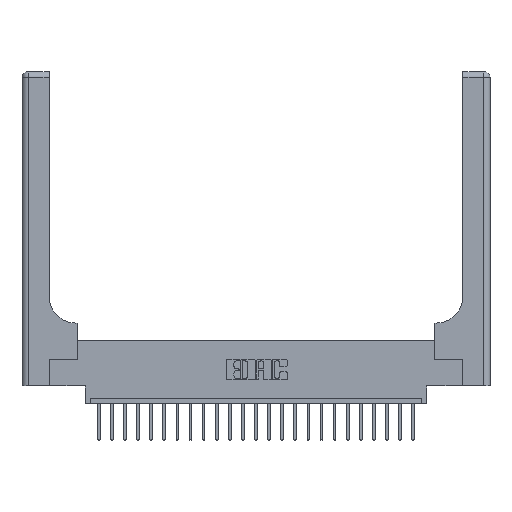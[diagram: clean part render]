
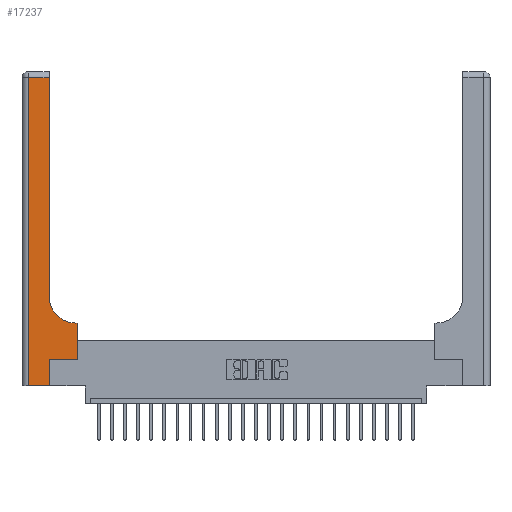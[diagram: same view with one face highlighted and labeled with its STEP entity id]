
A CAD part, top view. The second image highlights one B-rep face of the part: STEP entity #17237.
In plain terms, the highlighted planar face has unit normal (0, 0, 1).
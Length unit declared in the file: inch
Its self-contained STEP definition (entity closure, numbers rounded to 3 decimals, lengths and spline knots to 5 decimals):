
#562 = VERTEX_POINT ( 'NONE', #19831 ) ;
#1070 = DIRECTION ( 'NONE',  ( 0., 0., -1. ) ) ;
#1335 = DIRECTION ( 'NONE',  ( -1., 0., 0. ) ) ;
#1407 = CARTESIAN_POINT ( 'NONE',  ( 0.26, 0.85, 0.37 ) ) ;
#1485 = ORIENTED_EDGE ( 'NONE', *, *, #6124, .T. ) ;
#1580 = CARTESIAN_POINT ( 'NONE',  ( 0.06, 0., 0.37 ) ) ;
#2424 = CARTESIAN_POINT ( 'NONE',  ( 0.265, 0.25, 0.37 ) ) ;
#3102 = ORIENTED_EDGE ( 'NONE', *, *, #18087, .T. ) ;
#3321 = ORIENTED_EDGE ( 'NONE', *, *, #10830, .T. ) ;
#3739 = EDGE_CURVE ( 'NONE', #18704, #14132, #15753, .T. ) ;
#3836 = EDGE_CURVE ( 'NONE', #17118, #9090, #19285, .T. ) ;
#3995 = DIRECTION ( 'NONE',  ( 0., -1., 0. ) ) ;
#4008 = AXIS2_PLACEMENT_3D ( 'NONE', #20107, #22042, #14626 ) ;
#4789 = VECTOR ( 'NONE', #16347, 39.37008 ) ;
#5473 = AXIS2_PLACEMENT_3D ( 'NONE', #7974, #1070, #23013 ) ;
#6101 = LINE ( 'NONE', #2424, #14169 ) ;
#6124 = EDGE_CURVE ( 'NONE', #22109, #21624, #6384, .T. ) ;
#6230 = DIRECTION ( 'NONE',  ( 1., 0., 0. ) ) ;
#6342 = VECTOR ( 'NONE', #3995, 39.37008 ) ;
#6384 = LINE ( 'NONE', #13670, #18684 ) ;
#6736 = CARTESIAN_POINT ( 'NONE',  ( 0.265, 0.25, 0.37 ) ) ;
#6744 = ORIENTED_EDGE ( 'NONE', *, *, #3739, .T. ) ;
#6909 = CARTESIAN_POINT ( 'NONE',  ( 0.26, 0.6, 0.37 ) ) ;
#6923 = EDGE_CURVE ( 'NONE', #14132, #22109, #16586, .T. ) ;
#7754 = ORIENTED_EDGE ( 'NONE', *, *, #13706, .T. ) ;
#7974 = CARTESIAN_POINT ( 'NONE',  ( 0.51, 0.85, 0.37 ) ) ;
#8305 = EDGE_CURVE ( 'NONE', #21941, #18704, #8724, .T. ) ;
#8724 = LINE ( 'NONE', #6909, #14273 ) ;
#9090 = VERTEX_POINT ( 'NONE', #6736 ) ;
#9144 = CARTESIAN_POINT ( 'NONE',  ( 0.51, 0.6, 0.37 ) ) ;
#9542 = CARTESIAN_POINT ( 'NONE',  ( 0.06, 2.94, 0.37 ) ) ;
#9751 = CARTESIAN_POINT ( 'NONE',  ( 0.26, 2.94, 0.37 ) ) ;
#9886 = CARTESIAN_POINT ( 'NONE',  ( 0.265, 0., 0.37 ) ) ;
#10032 = EDGE_LOOP ( 'NONE', ( #19456, #1485, #23025, #3321, #22377, #7754, #3102, #10640, #6744 ) ) ;
#10592 = CARTESIAN_POINT ( 'NONE',  ( 0.265, 0., 0.37 ) ) ;
#10640 = ORIENTED_EDGE ( 'NONE', *, *, #8305, .T. ) ;
#10720 = VECTOR ( 'NONE', #20021, 39.37008 ) ;
#10830 = EDGE_CURVE ( 'NONE', #19618, #17118, #17869, .T. ) ;
#12540 = CARTESIAN_POINT ( 'NONE',  ( 0., 0., 0.37 ) ) ;
#12687 = CARTESIAN_POINT ( 'NONE',  ( 0.26, 3., 0.37 ) ) ;
#13046 = DIRECTION ( 'NONE',  ( 0., 1., 0. ) ) ;
#13089 = PLANE ( 'NONE',  #4008 ) ;
#13194 = LINE ( 'NONE', #16746, #6342 ) ;
#13577 = VECTOR ( 'NONE', #13046, 39.37008 ) ;
#13670 = CARTESIAN_POINT ( 'NONE',  ( 0., 2.94, 0.37 ) ) ;
#13706 = EDGE_CURVE ( 'NONE', #9090, #562, #6101, .T. ) ;
#14132 = VERTEX_POINT ( 'NONE', #1407 ) ;
#14169 = VECTOR ( 'NONE', #6230, 39.37008 ) ;
#14273 = VECTOR ( 'NONE', #1335, 39.37008 ) ;
#14626 = DIRECTION ( 'NONE',  ( -1., 0., 0. ) ) ;
#15094 = FACE_OUTER_BOUND ( 'NONE', #10032, .T. ) ;
#15165 = CARTESIAN_POINT ( 'NONE',  ( 0.528, 0.25, 0.37 ) ) ;
#15753 = CIRCLE ( 'NONE', #5473, 0.25 ) ;
#16347 = DIRECTION ( 'NONE',  ( 0., 1., 0. ) ) ;
#16586 = LINE ( 'NONE', #12687, #4789 ) ;
#16746 = CARTESIAN_POINT ( 'NONE',  ( 0.06, 3., 0.37 ) ) ;
#17118 = VERTEX_POINT ( 'NONE', #10592 ) ;
#17237 = ADVANCED_FACE ( 'NONE', ( #15094 ), #13089, .F. ) ;
#17869 = LINE ( 'NONE', #12540, #10720 ) ;
#18087 = EDGE_CURVE ( 'NONE', #562, #21941, #18854, .T. ) ;
#18684 = VECTOR ( 'NONE', #19123, 39.37008 ) ;
#18704 = VERTEX_POINT ( 'NONE', #9144 ) ;
#18724 = EDGE_CURVE ( 'NONE', #21624, #19618, #13194, .T. ) ;
#18854 = LINE ( 'NONE', #15165, #13577 ) ;
#19123 = DIRECTION ( 'NONE',  ( -1., 0., 0. ) ) ;
#19285 = LINE ( 'NONE', #9886, #21221 ) ;
#19456 = ORIENTED_EDGE ( 'NONE', *, *, #6923, .T. ) ;
#19618 = VERTEX_POINT ( 'NONE', #1580 ) ;
#19755 = DIRECTION ( 'NONE',  ( 0., 1., 0. ) ) ;
#19831 = CARTESIAN_POINT ( 'NONE',  ( 0.528, 0.25, 0.37 ) ) ;
#20021 = DIRECTION ( 'NONE',  ( 1., 0., 0. ) ) ;
#20107 = CARTESIAN_POINT ( 'NONE',  ( 0., 3., 0.37 ) ) ;
#21221 = VECTOR ( 'NONE', #19755, 39.37008 ) ;
#21624 = VERTEX_POINT ( 'NONE', #9542 ) ;
#21815 = CARTESIAN_POINT ( 'NONE',  ( 0.528, 0.6, 0.37 ) ) ;
#21941 = VERTEX_POINT ( 'NONE', #21815 ) ;
#22042 = DIRECTION ( 'NONE',  ( 0., 0., -1. ) ) ;
#22109 = VERTEX_POINT ( 'NONE', #9751 ) ;
#22377 = ORIENTED_EDGE ( 'NONE', *, *, #3836, .T. ) ;
#23013 = DIRECTION ( 'NONE',  ( 1., 0., 0. ) ) ;
#23025 = ORIENTED_EDGE ( 'NONE', *, *, #18724, .T. ) ;
